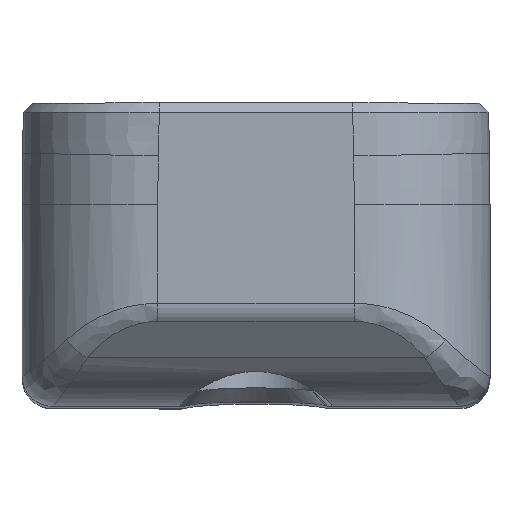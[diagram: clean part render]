
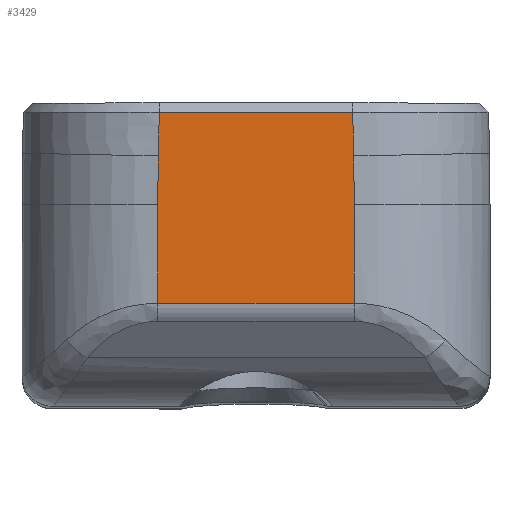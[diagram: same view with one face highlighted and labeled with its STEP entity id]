
A CAD part, top view. The second image highlights one B-rep face of the part: STEP entity #3429.
In plain terms, the highlighted planar face has unit normal (0, 0, 1).
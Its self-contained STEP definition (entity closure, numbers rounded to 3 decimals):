
#108=CIRCLE('',#3542,3191.507);
#326=CIRCLE('',#3846,156.5);
#327=CIRCLE('',#3847,156.5);
#328=CIRCLE('',#3848,3191.507);
#424=B_SPLINE_CURVE_WITH_KNOTS('',3,(#5158,#5159,#5160,#5161),
 .UNSPECIFIED.,.F.,.F.,(4,4),(-3.999,-3.998),
 .UNSPECIFIED.);
#430=B_SPLINE_CURVE_WITH_KNOTS('',3,(#5443,#5444,#5445,#5446),
 .UNSPECIFIED.,.F.,.F.,(4,4),(-1.334,-1.333),
 .UNSPECIFIED.);
#824=FACE_OUTER_BOUND('',#1076,.T.);
#1076=EDGE_LOOP('',(#2835,#2836,#2837,#2838,#2839,#2840,#2841,#2842,#2843,
#2844));
#1177=LINE('',#5138,#1293);
#1195=LINE('',#9249,#1311);
#1204=LINE('',#9733,#1320);
#1205=LINE('',#9738,#1321);
#1293=VECTOR('',#3962,10.);
#1311=VECTOR('',#4170,10.);
#1320=VECTOR('',#4603,10.);
#1321=VECTOR('',#4610,10.);
#1407=VERTEX_POINT('',#4966);
#1411=VERTEX_POINT('',#5135);
#1412=VERTEX_POINT('',#5137);
#1414=VERTEX_POINT('',#5270);
#1427=VERTEX_POINT('',#5511);
#1623=VERTEX_POINT('',#9239);
#1625=VERTEX_POINT('',#9245);
#1653=VERTEX_POINT('',#9732);
#1654=VERTEX_POINT('',#9737);
#1655=VERTEX_POINT('',#9739);
#1691=EDGE_CURVE('',#1411,#1412,#1177,.T.);
#1694=EDGE_CURVE('',#1412,#1407,#424,.T.);
#1706=EDGE_CURVE('',#1414,#1411,#430,.T.);
#1718=EDGE_CURVE('',#1427,#1414,#108,.T.);
#1927=EDGE_CURVE('',#1623,#1625,#1195,.T.);
#2089=EDGE_CURVE('',#1625,#1653,#1204,.T.);
#2091=EDGE_CURVE('',#1653,#1427,#326,.T.);
#2092=EDGE_CURVE('',#1654,#1623,#1205,.T.);
#2093=EDGE_CURVE('',#1655,#1654,#327,.T.);
#2094=EDGE_CURVE('',#1407,#1655,#328,.T.);
#2835=ORIENTED_EDGE('',*,*,#1706,.F.);
#2836=ORIENTED_EDGE('',*,*,#1718,.F.);
#2837=ORIENTED_EDGE('',*,*,#2091,.F.);
#2838=ORIENTED_EDGE('',*,*,#2089,.F.);
#2839=ORIENTED_EDGE('',*,*,#1927,.F.);
#2840=ORIENTED_EDGE('',*,*,#2092,.F.);
#2841=ORIENTED_EDGE('',*,*,#2093,.F.);
#2842=ORIENTED_EDGE('',*,*,#2094,.F.);
#2843=ORIENTED_EDGE('',*,*,#1694,.F.);
#2844=ORIENTED_EDGE('',*,*,#1691,.F.);
#3266=PLANE('',#3845);
#3429=ADVANCED_FACE('',(#824),#3266,.T.);
#3542=AXIS2_PLACEMENT_3D('',#5513,#3985,#3986);
#3845=AXIS2_PLACEMENT_3D('',#9735,#4606,#4607);
#3846=AXIS2_PLACEMENT_3D('',#9736,#4608,#4609);
#3847=AXIS2_PLACEMENT_3D('',#9740,#4611,#4612);
#3848=AXIS2_PLACEMENT_3D('',#9741,#4613,#4614);
#3962=DIRECTION('',(1.,0.,0.));
#3985=DIRECTION('center_axis',(0.,0.,1.));
#3986=DIRECTION('ref_axis',(1.,-0.004,0.));
#4170=DIRECTION('',(-1.,0.,0.));
#4603=DIRECTION('',(0.,1.,0.));
#4606=DIRECTION('center_axis',(0.,0.,1.));
#4607=DIRECTION('ref_axis',(0.,1.,0.));
#4608=DIRECTION('center_axis',(0.,0.,-1.));
#4609=DIRECTION('ref_axis',(-1.,0.01,0.));
#4610=DIRECTION('',(0.,-1.,0.));
#4611=DIRECTION('center_axis',(0.,0.,-1.));
#4612=DIRECTION('ref_axis',(1.,0.01,0.));
#4613=DIRECTION('center_axis',(0.,0.,1.));
#4614=DIRECTION('ref_axis',(-1.,-0.004,0.));
#4966=CARTESIAN_POINT('',(22.385,399.4,-120.588));
#5135=CARTESIAN_POINT('',(9.58,399.4,-120.588));
#5137=CARTESIAN_POINT('',(22.374,399.4,-120.588));
#5138=CARTESIAN_POINT('',(24.727,399.4,-120.588));
#5158=CARTESIAN_POINT('Ctrl Pts',(22.374,399.4,-120.588));
#5159=CARTESIAN_POINT('Ctrl Pts',(22.378,399.4,-120.588));
#5160=CARTESIAN_POINT('Ctrl Pts',(22.381,399.4,-120.588));
#5161=CARTESIAN_POINT('Ctrl Pts',(22.385,399.4,-120.588));
#5270=CARTESIAN_POINT('',(9.568,399.4,-120.588));
#5443=CARTESIAN_POINT('Ctrl Pts',(9.568,399.4,-120.588));
#5444=CARTESIAN_POINT('Ctrl Pts',(9.572,399.4,-120.588));
#5445=CARTESIAN_POINT('Ctrl Pts',(9.576,399.4,-120.588));
#5446=CARTESIAN_POINT('Ctrl Pts',(9.58,399.4,-120.588));
#5511=CARTESIAN_POINT('',(9.51,396.491,-120.588));
#5513=CARTESIAN_POINT('Origin',(-3181.326,461.945,-120.588));
#9239=CARTESIAN_POINT('',(22.477,386.732,-120.588));
#9245=CARTESIAN_POINT('',(9.477,386.732,-120.588));
#9249=CARTESIAN_POINT('',(32.477,386.732,-120.588));
#9732=CARTESIAN_POINT('',(9.477,393.281,-120.588));
#9733=CARTESIAN_POINT('',(9.477,420.5,-120.588));
#9735=CARTESIAN_POINT('Origin',(33.477,446.,-120.588));
#9736=CARTESIAN_POINT('Origin',(165.977,393.281,-120.588));
#9737=CARTESIAN_POINT('',(22.477,393.281,-120.588));
#9738=CARTESIAN_POINT('',(22.477,413.,-120.588));
#9739=CARTESIAN_POINT('',(22.444,396.491,-120.588));
#9740=CARTESIAN_POINT('Origin',(-134.023,393.281,-120.588));
#9741=CARTESIAN_POINT('Origin',(3213.279,461.945,-120.588));
